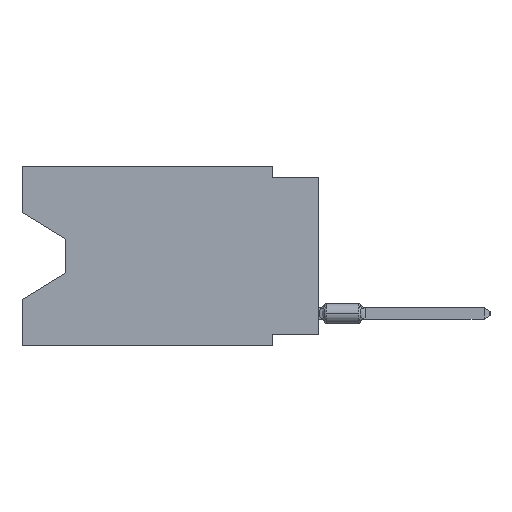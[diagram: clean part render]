
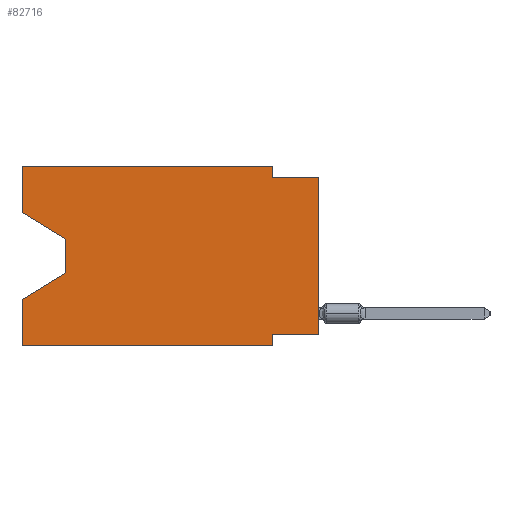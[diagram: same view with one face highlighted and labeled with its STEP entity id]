
A CAD part, left-side view. The second image highlights one B-rep face of the part: STEP entity #82716.
In plain terms, the highlighted planar face has unit normal (-1, 0, 0).
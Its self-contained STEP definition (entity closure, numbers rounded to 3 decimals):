
#129 = LINE ( 'NONE', #27718, #58683 ) ;
#1668 = ORIENTED_EDGE ( 'NONE', *, *, #35667, .T. ) ;
#4235 = CARTESIAN_POINT ( 'NONE',  ( 0., 16.383, 0. ) ) ;
#4494 = VECTOR ( 'NONE', #43356, 1000. ) ;
#5995 = EDGE_CURVE ( 'NONE', #20912, #63450, #81497, .T. ) ;
#7303 = EDGE_CURVE ( 'NONE', #23328, #65419, #86749, .T. ) ;
#7890 = LINE ( 'NONE', #35922, #31335 ) ;
#8911 = VECTOR ( 'NONE', #36924, 1000. ) ;
#9533 = DIRECTION ( 'NONE',  ( 0., 0., -1. ) ) ;
#10203 = CARTESIAN_POINT ( 'NONE',  ( 0., 16.383, -9.906 ) ) ;
#10918 = ORIENTED_EDGE ( 'NONE', *, *, #85838, .F. ) ;
#11804 = VECTOR ( 'NONE', #36465, 1000. ) ;
#12389 = ORIENTED_EDGE ( 'NONE', *, *, #49937, .F. ) ;
#13738 = DIRECTION ( 'NONE',  ( 0., 0., 1. ) ) ;
#13949 = CARTESIAN_POINT ( 'NONE',  ( 0., 2.54, -9.906 ) ) ;
#14062 = CARTESIAN_POINT ( 'NONE',  ( 0., 2.54, -9.271 ) ) ;
#16115 = DIRECTION ( 'NONE',  ( 0., -1., 0. ) ) ;
#16199 = CARTESIAN_POINT ( 'NONE',  ( 0., 0., -9.271 ) ) ;
#16626 = CARTESIAN_POINT ( 'NONE',  ( 0., 16.383, -2.546 ) ) ;
#16839 = EDGE_CURVE ( 'NONE', #27011, #65419, #70073, .T. ) ;
#16896 = CARTESIAN_POINT ( 'NONE',  ( 0., 13.97, -4.013 ) ) ;
#16905 = LINE ( 'NONE', #22692, #62427 ) ;
#18723 = CARTESIAN_POINT ( 'NONE',  ( 0., 2.54, -0.635 ) ) ;
#18953 = AXIS2_PLACEMENT_3D ( 'NONE', #23341, #77714, #9533 ) ;
#19820 = CARTESIAN_POINT ( 'NONE',  ( 0., 2.54, -9.906 ) ) ;
#20758 = DIRECTION ( 'NONE',  ( 0., 0., 1. ) ) ;
#20912 = VERTEX_POINT ( 'NONE', #16626 ) ;
#20976 = ORIENTED_EDGE ( 'NONE', *, *, #82385, .T. ) ;
#21870 = ORIENTED_EDGE ( 'NONE', *, *, #5995, .F. ) ;
#22692 = CARTESIAN_POINT ( 'NONE',  ( 0., 16.383, -2.546 ) ) ;
#22889 = LINE ( 'NONE', #16199, #4494 ) ;
#23117 = VECTOR ( 'NONE', #13738, 1000. ) ;
#23328 = VERTEX_POINT ( 'NONE', #34655 ) ;
#23341 = CARTESIAN_POINT ( 'NONE',  ( 0., 16.383, 0. ) ) ;
#24395 = VERTEX_POINT ( 'NONE', #27766 ) ;
#25134 = DIRECTION ( 'NONE',  ( 0., 0., -1. ) ) ;
#25136 = ORIENTED_EDGE ( 'NONE', *, *, #40062, .T. ) ;
#27011 = VERTEX_POINT ( 'NONE', #55266 ) ;
#27718 = CARTESIAN_POINT ( 'NONE',  ( 0., 0., 0. ) ) ;
#27766 = CARTESIAN_POINT ( 'NONE',  ( 0., 0., -0.635 ) ) ;
#28704 = FACE_OUTER_BOUND ( 'NONE', #59183, .T. ) ;
#29504 = DIRECTION ( 'NONE',  ( 0., 0.855, -0.519 ) ) ;
#30881 = ORIENTED_EDGE ( 'NONE', *, *, #7303, .F. ) ;
#31335 = VECTOR ( 'NONE', #35054, 1000. ) ;
#34655 = CARTESIAN_POINT ( 'NONE',  ( 0., 16.383, -9.906 ) ) ;
#35054 = DIRECTION ( 'NONE',  ( 0., -1., 0. ) ) ;
#35667 = EDGE_CURVE ( 'NONE', #20912, #70642, #16905, .T. ) ;
#35922 = CARTESIAN_POINT ( 'NONE',  ( 0., 16.383, 0. ) ) ;
#36465 = DIRECTION ( 'NONE',  ( 0., 0., -1. ) ) ;
#36924 = DIRECTION ( 'NONE',  ( 0., -1., 0. ) ) ;
#39266 = VERTEX_POINT ( 'NONE', #55968 ) ;
#40062 = EDGE_CURVE ( 'NONE', #39266, #24395, #129, .T. ) ;
#40945 = VECTOR ( 'NONE', #75940, 1000. ) ;
#41952 = CARTESIAN_POINT ( 'NONE',  ( 0., 0., -0.635 ) ) ;
#43356 = DIRECTION ( 'NONE',  ( 0., 1., 0. ) ) ;
#43933 = ORIENTED_EDGE ( 'NONE', *, *, #67534, .F. ) ;
#45479 = VERTEX_POINT ( 'NONE', #73283 ) ;
#46914 = DIRECTION ( 'NONE',  ( 0., 0., 1. ) ) ;
#47169 = VERTEX_POINT ( 'NONE', #18723 ) ;
#48749 = LINE ( 'NONE', #63417, #40945 ) ;
#49937 = EDGE_CURVE ( 'NONE', #45479, #47169, #48749, .T. ) ;
#55266 = CARTESIAN_POINT ( 'NONE',  ( 0., 13.97, -5.893 ) ) ;
#55968 = CARTESIAN_POINT ( 'NONE',  ( 0., 0., -9.271 ) ) ;
#56759 = PLANE ( 'NONE',  #18953 ) ;
#58683 = VECTOR ( 'NONE', #46914, 1000. ) ;
#59183 = EDGE_LOOP ( 'NONE', ( #1668, #65888, #61357, #30881, #20976, #10918, #43933, #25136, #65949, #12389, #82145, #21870 ) ) ;
#61357 = ORIENTED_EDGE ( 'NONE', *, *, #16839, .T. ) ;
#62364 = VECTOR ( 'NONE', #25134, 1000. ) ;
#62427 = VECTOR ( 'NONE', #71262, 1000. ) ;
#63367 = CARTESIAN_POINT ( 'NONE',  ( 0., 13.97, -5.893 ) ) ;
#63417 = CARTESIAN_POINT ( 'NONE',  ( 0., 2.54, 0. ) ) ;
#63450 = VERTEX_POINT ( 'NONE', #4235 ) ;
#65419 = VERTEX_POINT ( 'NONE', #75634 ) ;
#65888 = ORIENTED_EDGE ( 'NONE', *, *, #82409, .T. ) ;
#65949 = ORIENTED_EDGE ( 'NONE', *, *, #83035, .F. ) ;
#67534 = EDGE_CURVE ( 'NONE', #39266, #69672, #22889, .T. ) ;
#67791 = VECTOR ( 'NONE', #16115, 1000. ) ;
#68318 = CARTESIAN_POINT ( 'NONE',  ( 0., 13.97, -4.013 ) ) ;
#69672 = VERTEX_POINT ( 'NONE', #14062 ) ;
#70073 = LINE ( 'NONE', #63367, #82212 ) ;
#70642 = VERTEX_POINT ( 'NONE', #68318 ) ;
#71262 = DIRECTION ( 'NONE',  ( 0., -0.855, -0.519 ) ) ;
#73283 = CARTESIAN_POINT ( 'NONE',  ( 0., 2.54, 0. ) ) ;
#73464 = CARTESIAN_POINT ( 'NONE',  ( 0., 16.383, 0. ) ) ;
#74800 = VERTEX_POINT ( 'NONE', #13949 ) ;
#75634 = CARTESIAN_POINT ( 'NONE',  ( 0., 16.383, -7.36 ) ) ;
#75940 = DIRECTION ( 'NONE',  ( 0., 0., -1. ) ) ;
#76285 = LINE ( 'NONE', #41952, #67791 ) ;
#77714 = DIRECTION ( 'NONE',  ( 1., 0., 0. ) ) ;
#77927 = LINE ( 'NONE', #16896, #11804 ) ;
#78818 = LINE ( 'NONE', #10203, #8911 ) ;
#80055 = CARTESIAN_POINT ( 'NONE',  ( 0., 16.383, 0. ) ) ;
#80423 = VECTOR ( 'NONE', #20758, 1000. ) ;
#80841 = LINE ( 'NONE', #19820, #62364 ) ;
#81497 = LINE ( 'NONE', #73464, #23117 ) ;
#82145 = ORIENTED_EDGE ( 'NONE', *, *, #87920, .F. ) ;
#82212 = VECTOR ( 'NONE', #29504, 1000. ) ;
#82385 = EDGE_CURVE ( 'NONE', #23328, #74800, #78818, .T. ) ;
#82409 = EDGE_CURVE ( 'NONE', #70642, #27011, #77927, .T. ) ;
#82716 = ADVANCED_FACE ( 'NONE', ( #28704 ), #56759, .F. ) ;
#83035 = EDGE_CURVE ( 'NONE', #47169, #24395, #76285, .T. ) ;
#85838 = EDGE_CURVE ( 'NONE', #69672, #74800, #80841, .T. ) ;
#86749 = LINE ( 'NONE', #80055, #80423 ) ;
#87920 = EDGE_CURVE ( 'NONE', #63450, #45479, #7890, .T. ) ;
